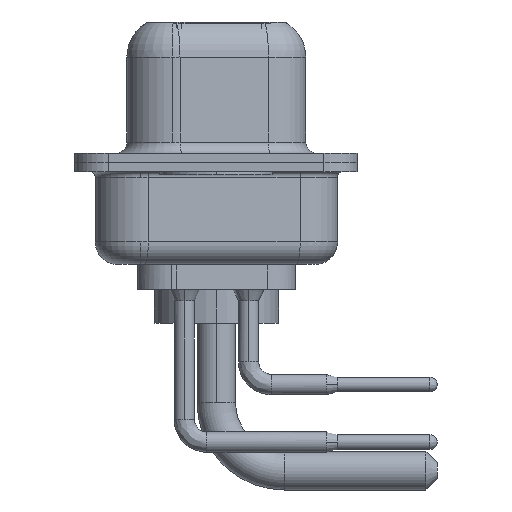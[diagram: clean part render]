
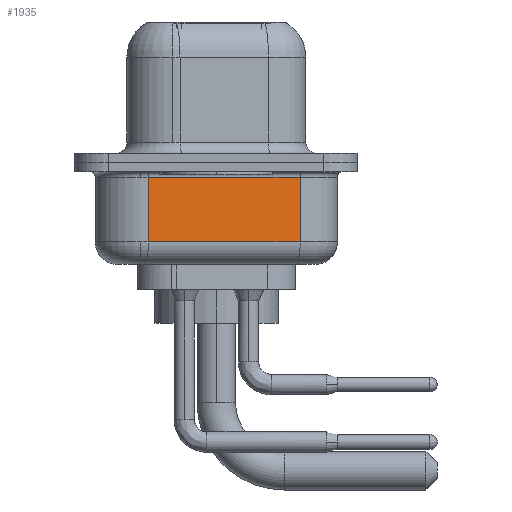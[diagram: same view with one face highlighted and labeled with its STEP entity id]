
A CAD part, left-side view. The second image highlights one B-rep face of the part: STEP entity #1935.
In plain terms, the highlighted planar face has unit normal (-0.985, -0.174, 0).
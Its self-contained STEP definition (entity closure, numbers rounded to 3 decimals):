
#54 = DIRECTION ( 'NONE',  ( 0.174, -0.985, 0. ) ) ;
#172 = EDGE_LOOP ( 'NONE', ( #10577, #5776, #11052, #6593 ) ) ;
#536 = EDGE_CURVE ( 'NONE', #5992, #7748, #14800, .T. ) ;
#1584 = VERTEX_POINT ( 'NONE', #16335 ) ;
#1935 = ADVANCED_FACE ( 'NONE', ( #5794 ), #5712, .F. ) ;
#2263 = VECTOR ( 'NONE', #54, 1000. ) ;
#2283 = LINE ( 'NONE', #10028, #4355 ) ;
#2502 = CARTESIAN_POINT ( 'NONE',  ( 4.062, -3.697, -0.65 ) ) ;
#3023 = CARTESIAN_POINT ( 'NONE',  ( 2.88, 3.003, -4.5 ) ) ;
#3410 = VERTEX_POINT ( 'NONE', #2502 ) ;
#3701 = VECTOR ( 'NONE', #3908, 1000. ) ;
#3851 = EDGE_CURVE ( 'NONE', #1584, #3410, #11503, .T. ) ;
#3908 = DIRECTION ( 'NONE',  ( 0., 0., 1. ) ) ;
#4355 = VECTOR ( 'NONE', #13892, 1000. ) ;
#5082 = CARTESIAN_POINT ( 'NONE',  ( 4.062, -3.697, -4.5 ) ) ;
#5712 = PLANE ( 'NONE',  #11230 ) ;
#5776 = ORIENTED_EDGE ( 'NONE', *, *, #15556, .T. ) ;
#5794 = FACE_OUTER_BOUND ( 'NONE', #172, .T. ) ;
#5992 = VERTEX_POINT ( 'NONE', #10304 ) ;
#6295 = CARTESIAN_POINT ( 'NONE',  ( 2.88, 3.003, -3.5 ) ) ;
#6593 = ORIENTED_EDGE ( 'NONE', *, *, #13841, .T. ) ;
#7748 = VERTEX_POINT ( 'NONE', #7840 ) ;
#7840 = CARTESIAN_POINT ( 'NONE',  ( 2.88, 3.003, -0.65 ) ) ;
#10012 = LINE ( 'NONE', #6295, #2263 ) ;
#10028 = CARTESIAN_POINT ( 'NONE',  ( 2.88, 3.003, -0.65 ) ) ;
#10304 = CARTESIAN_POINT ( 'NONE',  ( 2.88, 3.003, -3.5 ) ) ;
#10577 = ORIENTED_EDGE ( 'NONE', *, *, #536, .F. ) ;
#10861 = DIRECTION ( 'NONE',  ( 0., 0., 1. ) ) ;
#10867 = DIRECTION ( 'NONE',  ( 0.985, 0.174, 0. ) ) ;
#10913 = VECTOR ( 'NONE', #10861, 1000. ) ;
#11027 = CARTESIAN_POINT ( 'NONE',  ( 2.88, 3.003, -4.5 ) ) ;
#11052 = ORIENTED_EDGE ( 'NONE', *, *, #3851, .T. ) ;
#11230 = AXIS2_PLACEMENT_3D ( 'NONE', #11027, #10867, #16066 ) ;
#11503 = LINE ( 'NONE', #5082, #3701 ) ;
#13841 = EDGE_CURVE ( 'NONE', #3410, #7748, #2283, .T. ) ;
#13892 = DIRECTION ( 'NONE',  ( -0.174, 0.985, 0. ) ) ;
#14800 = LINE ( 'NONE', #3023, #10913 ) ;
#15556 = EDGE_CURVE ( 'NONE', #5992, #1584, #10012, .T. ) ;
#16066 = DIRECTION ( 'NONE',  ( -0.174, 0.985, 0. ) ) ;
#16335 = CARTESIAN_POINT ( 'NONE',  ( 4.062, -3.697, -3.5 ) ) ;
